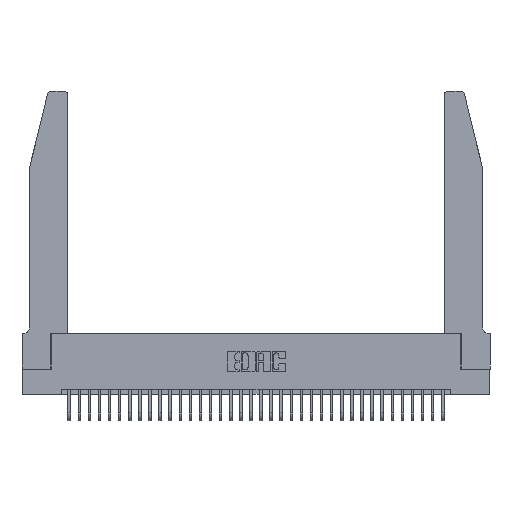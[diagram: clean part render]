
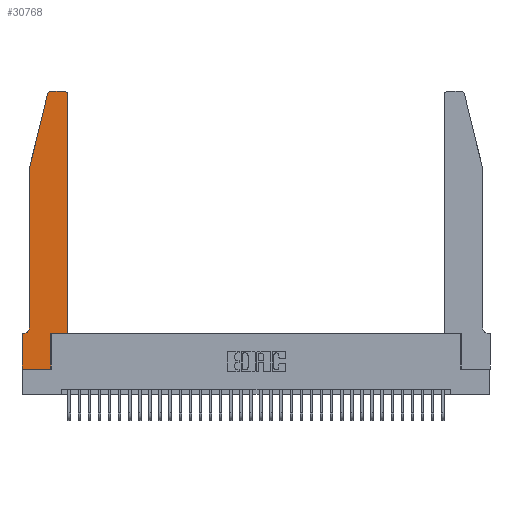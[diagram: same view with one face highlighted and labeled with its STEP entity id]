
A CAD part, top view. The second image highlights one B-rep face of the part: STEP entity #30768.
In plain terms, the highlighted planar face has unit normal (0, 0, 1).
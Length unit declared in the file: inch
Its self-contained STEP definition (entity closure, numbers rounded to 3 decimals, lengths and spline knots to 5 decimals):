
#394 = CARTESIAN_POINT ( 'NONE',  ( 0.2865, 0., 0.37 ) ) ;
#402 = EDGE_CURVE ( 'NONE', #20621, #14021, #9316, .T. ) ;
#487 = VECTOR ( 'NONE', #26360, 39.37008 ) ;
#756 = CARTESIAN_POINT ( 'NONE',  ( 0.0755, 2., 0.37 ) ) ;
#776 = VECTOR ( 'NONE', #5827, 39.37008 ) ;
#823 = DIRECTION ( 'NONE',  ( -1., 0., 0. ) ) ;
#844 = AXIS2_PLACEMENT_3D ( 'NONE', #13678, #32010, #16308 ) ;
#911 = CARTESIAN_POINT ( 'NONE',  ( 0., 0.35, 0.37 ) ) ;
#1426 = CARTESIAN_POINT ( 'NONE',  ( 0., 0., 0.37 ) ) ;
#1771 = CARTESIAN_POINT ( 'NONE',  ( 0.25487, 2.72718, 0.37 ) ) ;
#1776 = VERTEX_POINT ( 'NONE', #1928 ) ;
#1928 = CARTESIAN_POINT ( 'NONE',  ( 0.4505, 0.35, 0.37 ) ) ;
#2278 = ORIENTED_EDGE ( 'NONE', *, *, #21586, .T. ) ;
#2322 = AXIS2_PLACEMENT_3D ( 'NONE', #21250, #25112, #6799 ) ;
#2851 = CARTESIAN_POINT ( 'NONE',  ( 0., 0., 0.37 ) ) ;
#3197 = CARTESIAN_POINT ( 'NONE',  ( 0.4505, 0.35, 0.37 ) ) ;
#4144 = CARTESIAN_POINT ( 'NONE',  ( 0.4505, 2.72, 0.37 ) ) ;
#4182 = AXIS2_PLACEMENT_3D ( 'NONE', #22019, #6231, #24673 ) ;
#4745 = VECTOR ( 'NONE', #30154, 39.37008 ) ;
#4884 = EDGE_CURVE ( 'NONE', #10408, #20926, #8622, .T. ) ;
#4898 = EDGE_CURVE ( 'NONE', #18827, #1776, #21799, .T. ) ;
#5304 = FACE_OUTER_BOUND ( 'NONE', #19253, .T. ) ;
#5335 = EDGE_CURVE ( 'NONE', #1776, #10408, #8587, .T. ) ;
#5504 = CARTESIAN_POINT ( 'NONE',  ( 0.284, 2.75, 0.37 ) ) ;
#5560 = LINE ( 'NONE', #14339, #4745 ) ;
#5827 = DIRECTION ( 'NONE',  ( 1., 0., 0. ) ) ;
#6231 = DIRECTION ( 'NONE',  ( 0., 0., 1. ) ) ;
#6316 = VERTEX_POINT ( 'NONE', #911 ) ;
#6799 = DIRECTION ( 'NONE',  ( 1., 0., 0. ) ) ;
#7507 = LINE ( 'NONE', #21046, #487 ) ;
#7558 = CARTESIAN_POINT ( 'NONE',  ( 0.2865, 0.35, 0.37 ) ) ;
#7636 = VECTOR ( 'NONE', #15752, 39.37008 ) ;
#7960 = EDGE_CURVE ( 'NONE', #10746, #18758, #8465, .T. ) ;
#8465 = LINE ( 'NONE', #28838, #7636 ) ;
#8587 = LINE ( 'NONE', #28563, #21757 ) ;
#8622 = CIRCLE ( 'NONE', #844, 0.03 ) ;
#8808 = VECTOR ( 'NONE', #29911, 39.37008 ) ;
#9316 = CIRCLE ( 'NONE', #2322, 0.03 ) ;
#9684 = EDGE_CURVE ( 'NONE', #22678, #6316, #30558, .T. ) ;
#10408 = VERTEX_POINT ( 'NONE', #4144 ) ;
#10436 = ORIENTED_EDGE ( 'NONE', *, *, #402, .T. ) ;
#10468 = ORIENTED_EDGE ( 'NONE', *, *, #4884, .T. ) ;
#10710 = ORIENTED_EDGE ( 'NONE', *, *, #23792, .T. ) ;
#10746 = VERTEX_POINT ( 'NONE', #756 ) ;
#11256 = AXIS2_PLACEMENT_3D ( 'NONE', #32280, #16586, #823 ) ;
#11430 = PLANE ( 'NONE',  #4182 ) ;
#12683 = VECTOR ( 'NONE', #18471, 39.37008 ) ;
#13488 = LINE ( 'NONE', #28917, #12683 ) ;
#13678 = CARTESIAN_POINT ( 'NONE',  ( 0.4205, 2.72, 0.37 ) ) ;
#14021 = VERTEX_POINT ( 'NONE', #1771 ) ;
#14339 = CARTESIAN_POINT ( 'NONE',  ( 0.0755, 2., 0.37 ) ) ;
#15752 = DIRECTION ( 'NONE',  ( 0., -1., 0. ) ) ;
#16308 = DIRECTION ( 'NONE',  ( 1., 0., 0. ) ) ;
#16586 = DIRECTION ( 'NONE',  ( 0., 0., -1. ) ) ;
#17823 = EDGE_CURVE ( 'NONE', #26507, #19030, #7507, .T. ) ;
#18471 = DIRECTION ( 'NONE',  ( -1., 0., 0. ) ) ;
#18735 = ORIENTED_EDGE ( 'NONE', *, *, #21561, .T. ) ;
#18758 = VERTEX_POINT ( 'NONE', #23093 ) ;
#18827 = VERTEX_POINT ( 'NONE', #7558 ) ;
#19030 = VERTEX_POINT ( 'NONE', #394 ) ;
#19253 = EDGE_LOOP ( 'NONE', ( #28009, #10436, #18735, #20943, #10710, #22591, #2278, #28622, #24487, #21913, #27754, #10468 ) ) ;
#19763 = CARTESIAN_POINT ( 'NONE',  ( 0.4205, 2.75, 0.37 ) ) ;
#19837 = DIRECTION ( 'NONE',  ( 0., -1., 0. ) ) ;
#20611 = CIRCLE ( 'NONE', #11256, 0.07 ) ;
#20621 = VERTEX_POINT ( 'NONE', #5504 ) ;
#20926 = VERTEX_POINT ( 'NONE', #19763 ) ;
#20943 = ORIENTED_EDGE ( 'NONE', *, *, #7960, .T. ) ;
#21046 = CARTESIAN_POINT ( 'NONE',  ( 0., 0., 0.37 ) ) ;
#21250 = CARTESIAN_POINT ( 'NONE',  ( 0.284, 2.72, 0.37 ) ) ;
#21561 = EDGE_CURVE ( 'NONE', #14021, #10746, #5560, .T. ) ;
#21586 = EDGE_CURVE ( 'NONE', #6316, #26507, #24118, .T. ) ;
#21757 = VECTOR ( 'NONE', #31177, 39.37008 ) ;
#21799 = LINE ( 'NONE', #3197, #776 ) ;
#21913 = ORIENTED_EDGE ( 'NONE', *, *, #4898, .T. ) ;
#22019 = CARTESIAN_POINT ( 'NONE',  ( 0., 0.35, 0.37 ) ) ;
#22591 = ORIENTED_EDGE ( 'NONE', *, *, #9684, .T. ) ;
#22678 = VERTEX_POINT ( 'NONE', #27237 ) ;
#23093 = CARTESIAN_POINT ( 'NONE',  ( 0.0755, 0.42, 0.37 ) ) ;
#23792 = EDGE_CURVE ( 'NONE', #18758, #22678, #20611, .T. ) ;
#23975 = VECTOR ( 'NONE', #24113, 39.37008 ) ;
#24113 = DIRECTION ( 'NONE',  ( 0., 1., 0. ) ) ;
#24118 = LINE ( 'NONE', #1426, #31851 ) ;
#24487 = ORIENTED_EDGE ( 'NONE', *, *, #28789, .T. ) ;
#24673 = DIRECTION ( 'NONE',  ( 1., 0., 0. ) ) ;
#24884 = EDGE_CURVE ( 'NONE', #20926, #20621, #13488, .T. ) ;
#25112 = DIRECTION ( 'NONE',  ( 0., 0., 1. ) ) ;
#26360 = DIRECTION ( 'NONE',  ( 1., 0., 0. ) ) ;
#26507 = VERTEX_POINT ( 'NONE', #2851 ) ;
#27186 = CARTESIAN_POINT ( 'NONE',  ( 0.0755, 0.35, 0.37 ) ) ;
#27237 = CARTESIAN_POINT ( 'NONE',  ( 0.0055, 0.35, 0.37 ) ) ;
#27250 = LINE ( 'NONE', #29775, #23975 ) ;
#27754 = ORIENTED_EDGE ( 'NONE', *, *, #5335, .T. ) ;
#28009 = ORIENTED_EDGE ( 'NONE', *, *, #24884, .T. ) ;
#28563 = CARTESIAN_POINT ( 'NONE',  ( 0.4505, 0.35, 0.37 ) ) ;
#28622 = ORIENTED_EDGE ( 'NONE', *, *, #17823, .T. ) ;
#28789 = EDGE_CURVE ( 'NONE', #19030, #18827, #27250, .T. ) ;
#28838 = CARTESIAN_POINT ( 'NONE',  ( 0.0755, 2., 0.37 ) ) ;
#28917 = CARTESIAN_POINT ( 'NONE',  ( 0.2605, 2.75, 0.37 ) ) ;
#29775 = CARTESIAN_POINT ( 'NONE',  ( 0.2865, 0.35, 0.37 ) ) ;
#29911 = DIRECTION ( 'NONE',  ( -1., 0., 0. ) ) ;
#30154 = DIRECTION ( 'NONE',  ( -0.239, -0.971, 0. ) ) ;
#30558 = LINE ( 'NONE', #27186, #8808 ) ;
#30768 = ADVANCED_FACE ( 'NONE', ( #5304 ), #11430, .T. ) ;
#31177 = DIRECTION ( 'NONE',  ( 0., 1., 0. ) ) ;
#31851 = VECTOR ( 'NONE', #19837, 39.37008 ) ;
#32010 = DIRECTION ( 'NONE',  ( 0., 0., 1. ) ) ;
#32280 = CARTESIAN_POINT ( 'NONE',  ( 0.0055, 0.42, 0.37 ) ) ;
